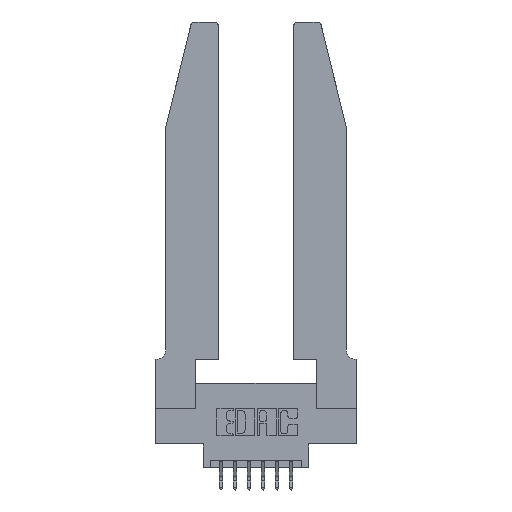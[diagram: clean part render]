
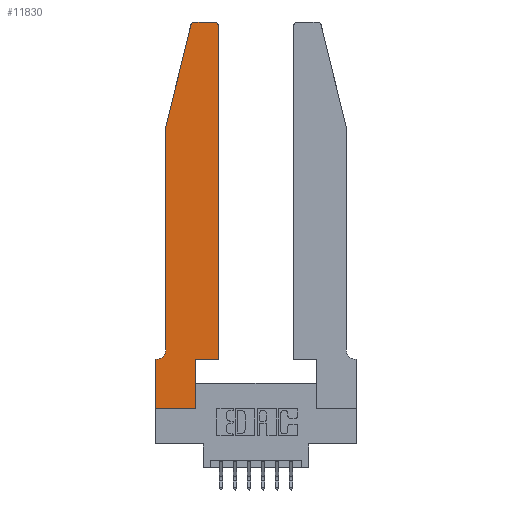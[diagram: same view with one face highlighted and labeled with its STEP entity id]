
A CAD part, top view. The second image highlights one B-rep face of the part: STEP entity #11830.
In plain terms, the highlighted planar face has unit normal (0, 0, 1).
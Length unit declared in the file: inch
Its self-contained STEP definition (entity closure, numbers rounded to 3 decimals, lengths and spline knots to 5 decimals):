
#170 = CARTESIAN_POINT ( 'NONE',  ( 0.284, 2.72, 0.37 ) ) ;
#183 = EDGE_CURVE ( 'NONE', #9946, #8794, #13239, .T. ) ;
#203 = DIRECTION ( 'NONE',  ( 0., 0., 1. ) ) ;
#299 = ORIENTED_EDGE ( 'NONE', *, *, #4424, .T. ) ;
#314 = CIRCLE ( 'NONE', #8230, 0.03 ) ;
#634 = AXIS2_PLACEMENT_3D ( 'NONE', #4561, #6673, #5502 ) ;
#909 = CARTESIAN_POINT ( 'NONE',  ( 0.0755, 2., 0.37 ) ) ;
#1345 = DIRECTION ( 'NONE',  ( 1., 0., 0. ) ) ;
#1434 = LINE ( 'NONE', #10863, #6891 ) ;
#1542 = EDGE_CURVE ( 'NONE', #8033, #13134, #9251, .T. ) ;
#1546 = ORIENTED_EDGE ( 'NONE', *, *, #1542, .T. ) ;
#1754 = VERTEX_POINT ( 'NONE', #11676 ) ;
#1904 = EDGE_CURVE ( 'NONE', #1931, #1754, #10335, .T. ) ;
#1931 = VERTEX_POINT ( 'NONE', #5725 ) ;
#2115 = CARTESIAN_POINT ( 'NONE',  ( 0.0755, 2., 0.37 ) ) ;
#2438 = CARTESIAN_POINT ( 'NONE',  ( 0.0055, 0.35, 0.37 ) ) ;
#2439 = EDGE_CURVE ( 'NONE', #5371, #13977, #13532, .T. ) ;
#2440 = DIRECTION ( 'NONE',  ( -1., 0., 0. ) ) ;
#2855 = DIRECTION ( 'NONE',  ( -1., 0., 0. ) ) ;
#2882 = DIRECTION ( 'NONE',  ( 0., 1., 0. ) ) ;
#2932 = CARTESIAN_POINT ( 'NONE',  ( 0.2865, 0.35, 0.37 ) ) ;
#2987 = ORIENTED_EDGE ( 'NONE', *, *, #11899, .T. ) ;
#3500 = ORIENTED_EDGE ( 'NONE', *, *, #1904, .T. ) ;
#3557 = VECTOR ( 'NONE', #2882, 39.37008 ) ;
#3594 = ORIENTED_EDGE ( 'NONE', *, *, #183, .T. ) ;
#3629 = AXIS2_PLACEMENT_3D ( 'NONE', #10392, #203, #13961 ) ;
#3657 = CARTESIAN_POINT ( 'NONE',  ( 0.0755, 2., 0.37 ) ) ;
#3667 = PLANE ( 'NONE',  #3629 ) ;
#3772 = CARTESIAN_POINT ( 'NONE',  ( 0.0755, 0.35, 0.37 ) ) ;
#3887 = DIRECTION ( 'NONE',  ( 1., 0., 0. ) ) ;
#3976 = VECTOR ( 'NONE', #2440, 39.37008 ) ;
#4045 = CARTESIAN_POINT ( 'NONE',  ( 0.4505, 2.72, 0.37 ) ) ;
#4424 = EDGE_CURVE ( 'NONE', #5072, #4430, #9907, .T. ) ;
#4430 = VERTEX_POINT ( 'NONE', #2438 ) ;
#4561 = CARTESIAN_POINT ( 'NONE',  ( 0.4205, 2.72, 0.37 ) ) ;
#4654 = CARTESIAN_POINT ( 'NONE',  ( 0.284, 2.75, 0.37 ) ) ;
#4794 = EDGE_CURVE ( 'NONE', #13977, #5898, #13632, .T. ) ;
#5022 = CARTESIAN_POINT ( 'NONE',  ( 0.4505, 0.35, 0.37 ) ) ;
#5072 = VERTEX_POINT ( 'NONE', #12431 ) ;
#5232 = LINE ( 'NONE', #12623, #8240 ) ;
#5371 = VERTEX_POINT ( 'NONE', #8853 ) ;
#5502 = DIRECTION ( 'NONE',  ( 1., 0., 0. ) ) ;
#5725 = CARTESIAN_POINT ( 'NONE',  ( 0., 0.35, 0.37 ) ) ;
#5738 = LINE ( 'NONE', #3772, #3976 ) ;
#5863 = ORIENTED_EDGE ( 'NONE', *, *, #4794, .T. ) ;
#5898 = VERTEX_POINT ( 'NONE', #13572 ) ;
#6029 = EDGE_LOOP ( 'NONE', ( #11527, #10005, #3594, #13078, #299, #2987, #3500, #7474, #1546, #13695, #6634, #5863 ) ) ;
#6164 = EDGE_CURVE ( 'NONE', #14176, #9946, #314, .T. ) ;
#6250 = VECTOR ( 'NONE', #14330, 39.37008 ) ;
#6252 = EDGE_CURVE ( 'NONE', #1754, #8033, #5232, .T. ) ;
#6634 = ORIENTED_EDGE ( 'NONE', *, *, #2439, .T. ) ;
#6673 = DIRECTION ( 'NONE',  ( 0., 0., 1. ) ) ;
#6839 = CARTESIAN_POINT ( 'NONE',  ( 0.2865, 0., 0.37 ) ) ;
#6891 = VECTOR ( 'NONE', #2855, 39.37008 ) ;
#6947 = AXIS2_PLACEMENT_3D ( 'NONE', #9414, #8084, #13815 ) ;
#7474 = ORIENTED_EDGE ( 'NONE', *, *, #6252, .T. ) ;
#7798 = LINE ( 'NONE', #2115, #13136 ) ;
#8033 = VERTEX_POINT ( 'NONE', #6839 ) ;
#8056 = DIRECTION ( 'NONE',  ( 0., 0., 1. ) ) ;
#8084 = DIRECTION ( 'NONE',  ( 0., 0., -1. ) ) ;
#8230 = AXIS2_PLACEMENT_3D ( 'NONE', #170, #8056, #8389 ) ;
#8240 = VECTOR ( 'NONE', #1345, 39.37008 ) ;
#8389 = DIRECTION ( 'NONE',  ( 1., 0., 0. ) ) ;
#8713 = VECTOR ( 'NONE', #3887, 39.37008 ) ;
#8794 = VERTEX_POINT ( 'NONE', #909 ) ;
#8853 = CARTESIAN_POINT ( 'NONE',  ( 0.4505, 0.35, 0.37 ) ) ;
#9164 = CARTESIAN_POINT ( 'NONE',  ( 0.2865, 0.35, 0.37 ) ) ;
#9251 = LINE ( 'NONE', #2932, #6250 ) ;
#9414 = CARTESIAN_POINT ( 'NONE',  ( 0.0055, 0.42, 0.37 ) ) ;
#9907 = CIRCLE ( 'NONE', #6947, 0.07 ) ;
#9946 = VERTEX_POINT ( 'NONE', #10364 ) ;
#10005 = ORIENTED_EDGE ( 'NONE', *, *, #6164, .T. ) ;
#10156 = VECTOR ( 'NONE', #13636, 39.37008 ) ;
#10335 = LINE ( 'NONE', #12535, #10156 ) ;
#10358 = EDGE_CURVE ( 'NONE', #8794, #5072, #7798, .T. ) ;
#10364 = CARTESIAN_POINT ( 'NONE',  ( 0.25487, 2.72718, 0.37 ) ) ;
#10392 = CARTESIAN_POINT ( 'NONE',  ( 0., 0.35, 0.37 ) ) ;
#10837 = EDGE_CURVE ( 'NONE', #5898, #14176, #1434, .T. ) ;
#10863 = CARTESIAN_POINT ( 'NONE',  ( 0.2605, 2.75, 0.37 ) ) ;
#11527 = ORIENTED_EDGE ( 'NONE', *, *, #10837, .T. ) ;
#11596 = DIRECTION ( 'NONE',  ( -0.239, -0.971, 0. ) ) ;
#11676 = CARTESIAN_POINT ( 'NONE',  ( 0., 0., 0.37 ) ) ;
#11751 = LINE ( 'NONE', #5022, #8713 ) ;
#11830 = ADVANCED_FACE ( 'NONE', ( #13029 ), #3667, .T. ) ;
#11899 = EDGE_CURVE ( 'NONE', #4430, #1931, #5738, .T. ) ;
#12280 = DIRECTION ( 'NONE',  ( 0., -1., 0. ) ) ;
#12431 = CARTESIAN_POINT ( 'NONE',  ( 0.0755, 0.42, 0.37 ) ) ;
#12535 = CARTESIAN_POINT ( 'NONE',  ( 0., 0., 0.37 ) ) ;
#12623 = CARTESIAN_POINT ( 'NONE',  ( 0., 0., 0.37 ) ) ;
#13029 = FACE_OUTER_BOUND ( 'NONE', #6029, .T. ) ;
#13078 = ORIENTED_EDGE ( 'NONE', *, *, #10358, .T. ) ;
#13134 = VERTEX_POINT ( 'NONE', #9164 ) ;
#13136 = VECTOR ( 'NONE', #12280, 39.37008 ) ;
#13239 = LINE ( 'NONE', #3657, #13422 ) ;
#13422 = VECTOR ( 'NONE', #11596, 39.37008 ) ;
#13532 = LINE ( 'NONE', #14126, #3557 ) ;
#13572 = CARTESIAN_POINT ( 'NONE',  ( 0.4205, 2.75, 0.37 ) ) ;
#13632 = CIRCLE ( 'NONE', #634, 0.03 ) ;
#13636 = DIRECTION ( 'NONE',  ( 0., -1., 0. ) ) ;
#13695 = ORIENTED_EDGE ( 'NONE', *, *, #14365, .T. ) ;
#13815 = DIRECTION ( 'NONE',  ( -1., 0., 0. ) ) ;
#13961 = DIRECTION ( 'NONE',  ( 1., 0., 0. ) ) ;
#13977 = VERTEX_POINT ( 'NONE', #4045 ) ;
#14126 = CARTESIAN_POINT ( 'NONE',  ( 0.4505, 0.35, 0.37 ) ) ;
#14176 = VERTEX_POINT ( 'NONE', #4654 ) ;
#14330 = DIRECTION ( 'NONE',  ( 0., 1., 0. ) ) ;
#14365 = EDGE_CURVE ( 'NONE', #13134, #5371, #11751, .T. ) ;
